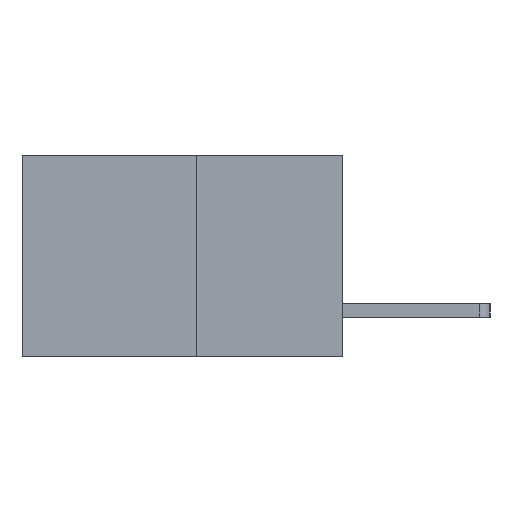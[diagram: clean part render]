
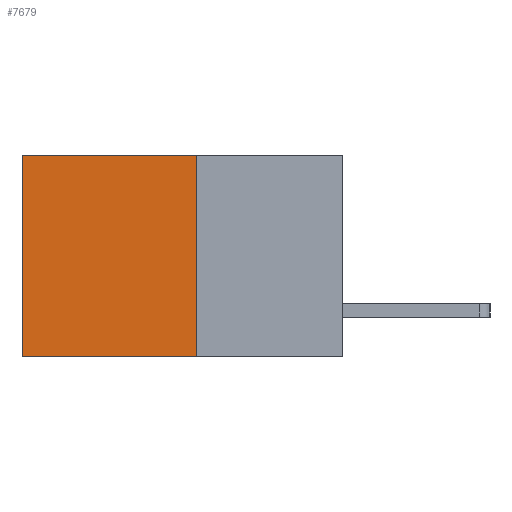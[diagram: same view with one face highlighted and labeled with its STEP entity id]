
A CAD part, left-side view. The second image highlights one B-rep face of the part: STEP entity #7679.
In plain terms, the highlighted planar face has unit normal (-1, 0, 0).
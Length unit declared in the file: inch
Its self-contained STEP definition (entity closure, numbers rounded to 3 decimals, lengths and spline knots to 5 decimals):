
#231 = EDGE_LOOP ( 'NONE', ( #6950, #1788, #1275, #8509 ) ) ;
#801 = PLANE ( 'NONE',  #4775 ) ;
#998 = VECTOR ( 'NONE', #5301, 39.37008 ) ;
#1026 = LINE ( 'NONE', #8607, #8304 ) ;
#1261 = DIRECTION ( 'NONE',  ( 1., 0., 0. ) ) ;
#1275 = ORIENTED_EDGE ( 'NONE', *, *, #1440, .F. ) ;
#1440 = EDGE_CURVE ( 'NONE', #1474, #6618, #4218, .T. ) ;
#1474 = VERTEX_POINT ( 'NONE', #4280 ) ;
#1571 = LINE ( 'NONE', #4936, #5159 ) ;
#1788 = ORIENTED_EDGE ( 'NONE', *, *, #5745, .F. ) ;
#2769 = CARTESIAN_POINT ( 'NONE',  ( 0.277, 0.27, -0.37 ) ) ;
#2792 = DIRECTION ( 'NONE',  ( 0., 0., -1. ) ) ;
#3276 = CARTESIAN_POINT ( 'NONE',  ( 0.277, 0.27, -0.37 ) ) ;
#3451 = FACE_OUTER_BOUND ( 'NONE', #231, .T. ) ;
#3612 = CARTESIAN_POINT ( 'NONE',  ( 0.277, 0.27, -0.37 ) ) ;
#3719 = VERTEX_POINT ( 'NONE', #6516 ) ;
#4058 = CARTESIAN_POINT ( 'NONE',  ( 0.277, 0.59, 0. ) ) ;
#4218 = LINE ( 'NONE', #2769, #7742 ) ;
#4280 = CARTESIAN_POINT ( 'NONE',  ( 0.277, 0.27, 0. ) ) ;
#4407 = DIRECTION ( 'NONE',  ( 0., 0., -1. ) ) ;
#4604 = EDGE_CURVE ( 'NONE', #4952, #3719, #1026, .T. ) ;
#4775 = AXIS2_PLACEMENT_3D ( 'NONE', #3276, #1261, #4407 ) ;
#4936 = CARTESIAN_POINT ( 'NONE',  ( 0.277, 0.27, -0.37 ) ) ;
#4952 = VERTEX_POINT ( 'NONE', #4058 ) ;
#5159 = VECTOR ( 'NONE', #6656, 39.37008 ) ;
#5289 = CARTESIAN_POINT ( 'NONE',  ( 0.277, 0.27, 0. ) ) ;
#5301 = DIRECTION ( 'NONE',  ( 0., 1., 0. ) ) ;
#5745 = EDGE_CURVE ( 'NONE', #6618, #3719, #1571, .T. ) ;
#6043 = EDGE_CURVE ( 'NONE', #1474, #4952, #6725, .T. ) ;
#6516 = CARTESIAN_POINT ( 'NONE',  ( 0.277, 0.59, -0.37 ) ) ;
#6618 = VERTEX_POINT ( 'NONE', #3612 ) ;
#6656 = DIRECTION ( 'NONE',  ( 0., 1., 0. ) ) ;
#6725 = LINE ( 'NONE', #5289, #998 ) ;
#6950 = ORIENTED_EDGE ( 'NONE', *, *, #4604, .T. ) ;
#7654 = DIRECTION ( 'NONE',  ( 0., 0., -1. ) ) ;
#7679 = ADVANCED_FACE ( 'NONE', ( #3451 ), #801, .F. ) ;
#7742 = VECTOR ( 'NONE', #2792, 39.37008 ) ;
#8304 = VECTOR ( 'NONE', #7654, 39.37008 ) ;
#8509 = ORIENTED_EDGE ( 'NONE', *, *, #6043, .T. ) ;
#8607 = CARTESIAN_POINT ( 'NONE',  ( 0.277, 0.59, -0.37 ) ) ;
